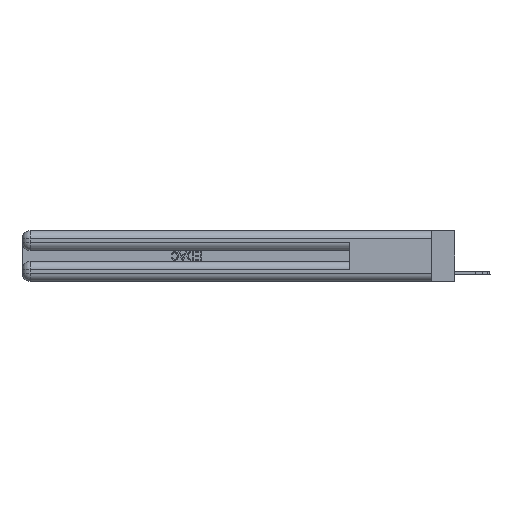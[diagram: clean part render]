
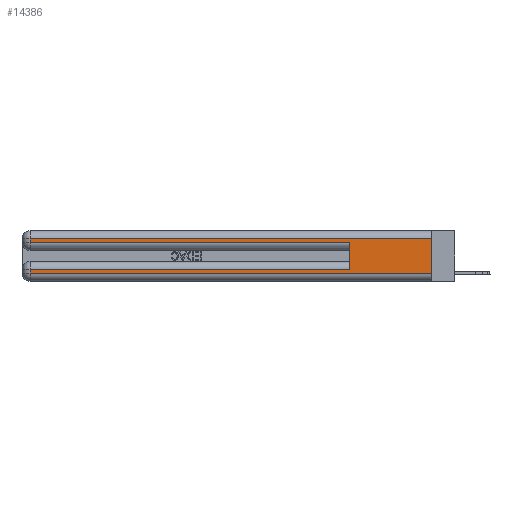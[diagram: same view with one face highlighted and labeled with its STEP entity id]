
A CAD part, left-side view. The second image highlights one B-rep face of the part: STEP entity #14386.
In plain terms, the highlighted planar face has unit normal (-1, 0, 0).
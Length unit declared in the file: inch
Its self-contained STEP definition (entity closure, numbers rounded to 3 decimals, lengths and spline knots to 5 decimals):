
#91 = DIRECTION ( 'NONE',  ( 0., 0., -1. ) ) ;
#114 = EDGE_CURVE ( 'NONE', #13570, #13623, #20397, .T. ) ;
#321 = DIRECTION ( 'NONE',  ( 0., -1., 0. ) ) ;
#400 = CARTESIAN_POINT ( 'NONE',  ( 0., 0., 0.37 ) ) ;
#827 = AXIS2_PLACEMENT_3D ( 'NONE', #18499, #23001, #9677 ) ;
#1344 = ORIENTED_EDGE ( 'NONE', *, *, #27973, .T. ) ;
#1824 = EDGE_CURVE ( 'NONE', #8348, #22992, #5096, .T. ) ;
#4272 = ORIENTED_EDGE ( 'NONE', *, *, #114, .F. ) ;
#4710 = LINE ( 'NONE', #6592, #17714 ) ;
#5096 = LINE ( 'NONE', #21141, #17373 ) ;
#5194 = VERTEX_POINT ( 'NONE', #6911 ) ;
#5299 = VERTEX_POINT ( 'NONE', #16084 ) ;
#5452 = VERTEX_POINT ( 'NONE', #17239 ) ;
#6008 = VECTOR ( 'NONE', #91, 39.37008 ) ;
#6019 = CARTESIAN_POINT ( 'NONE',  ( 0., 0., 0.06 ) ) ;
#6114 = ORIENTED_EDGE ( 'NONE', *, *, #24454, .T. ) ;
#6173 = CARTESIAN_POINT ( 'NONE',  ( 0., 2.94, 0.085 ) ) ;
#6440 = DIRECTION ( 'NONE',  ( 0., -1., 0. ) ) ;
#6592 = CARTESIAN_POINT ( 'NONE',  ( 0., 0., 0.31 ) ) ;
#6871 = LINE ( 'NONE', #20321, #23952 ) ;
#6885 = VECTOR ( 'NONE', #6440, 39.37008 ) ;
#6911 = CARTESIAN_POINT ( 'NONE',  ( 0., 2.94, 0.285 ) ) ;
#8348 = VERTEX_POINT ( 'NONE', #6173 ) ;
#8923 = DIRECTION ( 'NONE',  ( 0., 1., 0. ) ) ;
#8969 = LINE ( 'NONE', #11593, #23101 ) ;
#9677 = DIRECTION ( 'NONE',  ( 0., 0., -1. ) ) ;
#10970 = LINE ( 'NONE', #26482, #28400 ) ;
#11080 = EDGE_CURVE ( 'NONE', #22992, #13623, #24139, .T. ) ;
#11593 = CARTESIAN_POINT ( 'NONE',  ( 0., 0.6, 0.145 ) ) ;
#11993 = ORIENTED_EDGE ( 'NONE', *, *, #22890, .T. ) ;
#12339 = EDGE_CURVE ( 'NONE', #15556, #5194, #20355, .T. ) ;
#13210 = CARTESIAN_POINT ( 'NONE',  ( 0., 0., 0.31 ) ) ;
#13570 = VERTEX_POINT ( 'NONE', #13210 ) ;
#13623 = VERTEX_POINT ( 'NONE', #26680 ) ;
#14186 = CARTESIAN_POINT ( 'NONE',  ( 0., 2.94, 0.06 ) ) ;
#14386 = ADVANCED_FACE ( 'NONE', ( #22854 ), #18349, .F. ) ;
#14451 = DIRECTION ( 'NONE',  ( 0., 0., -1. ) ) ;
#15556 = VERTEX_POINT ( 'NONE', #16707 ) ;
#16084 = CARTESIAN_POINT ( 'NONE',  ( 0., 0.6, 0.085 ) ) ;
#16707 = CARTESIAN_POINT ( 'NONE',  ( 0., 2.94, 0.31 ) ) ;
#17239 = CARTESIAN_POINT ( 'NONE',  ( 0., 0.6, 0.285 ) ) ;
#17373 = VECTOR ( 'NONE', #14451, 39.37008 ) ;
#17714 = VECTOR ( 'NONE', #21949, 39.37008 ) ;
#17894 = DIRECTION ( 'NONE',  ( 0., 0., 1. ) ) ;
#18349 = PLANE ( 'NONE',  #827 ) ;
#18499 = CARTESIAN_POINT ( 'NONE',  ( 0., 0., 0.37 ) ) ;
#19706 = ORIENTED_EDGE ( 'NONE', *, *, #21888, .F. ) ;
#20080 = CARTESIAN_POINT ( 'NONE',  ( 0., 2.94, 0.37 ) ) ;
#20321 = CARTESIAN_POINT ( 'NONE',  ( 0., 0., 0.285 ) ) ;
#20355 = LINE ( 'NONE', #20080, #6008 ) ;
#20397 = LINE ( 'NONE', #400, #21161 ) ;
#21141 = CARTESIAN_POINT ( 'NONE',  ( 0., 2.94, 0.37 ) ) ;
#21161 = VECTOR ( 'NONE', #26407, 39.37008 ) ;
#21888 = EDGE_CURVE ( 'NONE', #5299, #5452, #8969, .T. ) ;
#21949 = DIRECTION ( 'NONE',  ( 0., 1., 0. ) ) ;
#22854 = FACE_OUTER_BOUND ( 'NONE', #25323, .T. ) ;
#22890 = EDGE_CURVE ( 'NONE', #5299, #8348, #10970, .T. ) ;
#22992 = VERTEX_POINT ( 'NONE', #14186 ) ;
#23001 = DIRECTION ( 'NONE',  ( 1., 0., 0. ) ) ;
#23101 = VECTOR ( 'NONE', #17894, 39.37008 ) ;
#23398 = ORIENTED_EDGE ( 'NONE', *, *, #11080, .T. ) ;
#23952 = VECTOR ( 'NONE', #321, 39.37008 ) ;
#23964 = ORIENTED_EDGE ( 'NONE', *, *, #12339, .T. ) ;
#24139 = LINE ( 'NONE', #6019, #6885 ) ;
#24454 = EDGE_CURVE ( 'NONE', #13570, #15556, #4710, .T. ) ;
#25323 = EDGE_LOOP ( 'NONE', ( #4272, #6114, #23964, #1344, #19706, #11993, #26699, #23398 ) ) ;
#26407 = DIRECTION ( 'NONE',  ( 0., 0., -1. ) ) ;
#26482 = CARTESIAN_POINT ( 'NONE',  ( 0., 0., 0.085 ) ) ;
#26680 = CARTESIAN_POINT ( 'NONE',  ( 0., 0., 0.06 ) ) ;
#26699 = ORIENTED_EDGE ( 'NONE', *, *, #1824, .T. ) ;
#27973 = EDGE_CURVE ( 'NONE', #5194, #5452, #6871, .T. ) ;
#28400 = VECTOR ( 'NONE', #8923, 39.37008 ) ;
